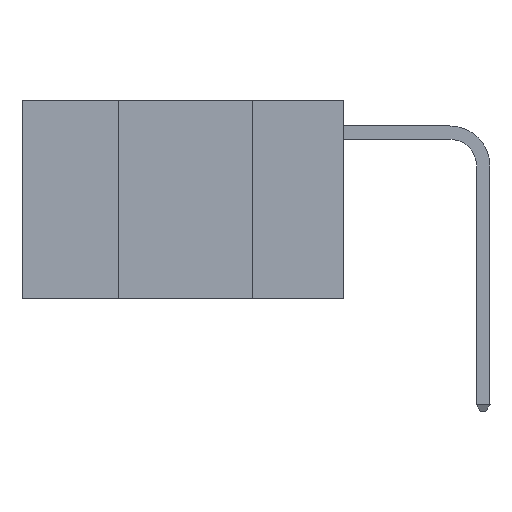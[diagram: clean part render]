
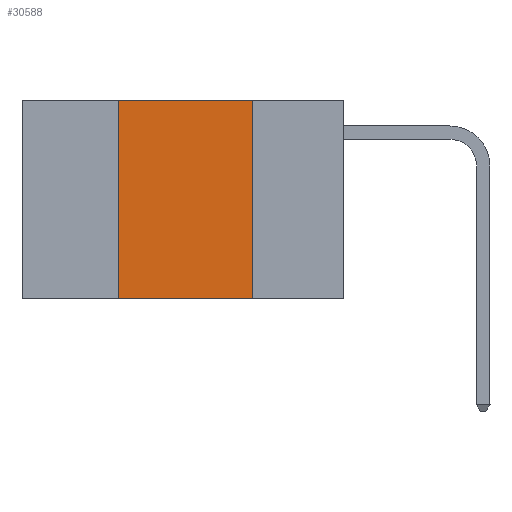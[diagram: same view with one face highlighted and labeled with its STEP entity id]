
A CAD part, left-side view. The second image highlights one B-rep face of the part: STEP entity #30588.
In plain terms, the highlighted planar face has unit normal (-1, 0, 0).
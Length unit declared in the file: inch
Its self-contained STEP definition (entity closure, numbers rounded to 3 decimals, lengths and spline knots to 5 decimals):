
#610 = CARTESIAN_POINT ( 'NONE',  ( 0., 0.6, -0.37 ) ) ;
#661 = LINE ( 'NONE', #14324, #13587 ) ;
#763 = CARTESIAN_POINT ( 'NONE',  ( 0., 0.17, 0. ) ) ;
#3244 = DIRECTION ( 'NONE',  ( 0., 0., -1. ) ) ;
#3301 = DIRECTION ( 'NONE',  ( 0., 0., -1. ) ) ;
#3351 = LINE ( 'NONE', #12835, #10573 ) ;
#5227 = VERTEX_POINT ( 'NONE', #6541 ) ;
#6541 = CARTESIAN_POINT ( 'NONE',  ( 0., 0.17, -0.37 ) ) ;
#7209 = EDGE_CURVE ( 'NONE', #12499, #29800, #3351, .T. ) ;
#8636 = VERTEX_POINT ( 'NONE', #27734 ) ;
#10573 = VECTOR ( 'NONE', #26993, 39.37008 ) ;
#12499 = VERTEX_POINT ( 'NONE', #12766 ) ;
#12766 = CARTESIAN_POINT ( 'NONE',  ( 0., 0.42, -0.37 ) ) ;
#12835 = CARTESIAN_POINT ( 'NONE',  ( 0., 0.42, 0. ) ) ;
#13587 = VECTOR ( 'NONE', #23828, 39.37008 ) ;
#14324 = CARTESIAN_POINT ( 'NONE',  ( 0., 0.6, 0. ) ) ;
#15406 = PLANE ( 'NONE',  #18692 ) ;
#17797 = DIRECTION ( 'NONE',  ( 1., 0., 0. ) ) ;
#18380 = LINE ( 'NONE', #610, #30022 ) ;
#18692 = AXIS2_PLACEMENT_3D ( 'NONE', #24668, #17797, #3301 ) ;
#18904 = LINE ( 'NONE', #763, #30542 ) ;
#20034 = ORIENTED_EDGE ( 'NONE', *, *, #24787, .F. ) ;
#20263 = ORIENTED_EDGE ( 'NONE', *, *, #25855, .F. ) ;
#20292 = ORIENTED_EDGE ( 'NONE', *, *, #7209, .F. ) ;
#20375 = ORIENTED_EDGE ( 'NONE', *, *, #20681, .T. ) ;
#20681 = EDGE_CURVE ( 'NONE', #12499, #5227, #18380, .T. ) ;
#22206 = DIRECTION ( 'NONE',  ( 0., -1., 0. ) ) ;
#22281 = EDGE_LOOP ( 'NONE', ( #20034, #20263, #20292, #20375 ) ) ;
#22580 = FACE_OUTER_BOUND ( 'NONE', #22281, .T. ) ;
#23828 = DIRECTION ( 'NONE',  ( 0., -1., 0. ) ) ;
#24668 = CARTESIAN_POINT ( 'NONE',  ( 0., 0.6, 0. ) ) ;
#24787 = EDGE_CURVE ( 'NONE', #8636, #5227, #18904, .T. ) ;
#25855 = EDGE_CURVE ( 'NONE', #29800, #8636, #661, .T. ) ;
#26993 = DIRECTION ( 'NONE',  ( 0., 0., 1. ) ) ;
#27734 = CARTESIAN_POINT ( 'NONE',  ( 0., 0.17, 0. ) ) ;
#29800 = VERTEX_POINT ( 'NONE', #29974 ) ;
#29974 = CARTESIAN_POINT ( 'NONE',  ( 0., 0.42, 0. ) ) ;
#30022 = VECTOR ( 'NONE', #22206, 39.37008 ) ;
#30542 = VECTOR ( 'NONE', #3244, 39.37008 ) ;
#30588 = ADVANCED_FACE ( 'NONE', ( #22580 ), #15406, .F. ) ;
